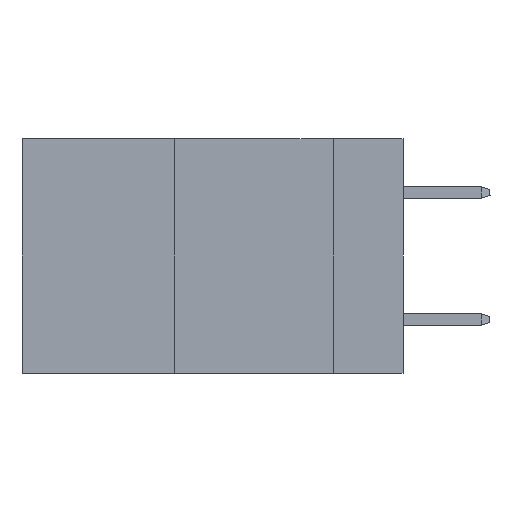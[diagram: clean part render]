
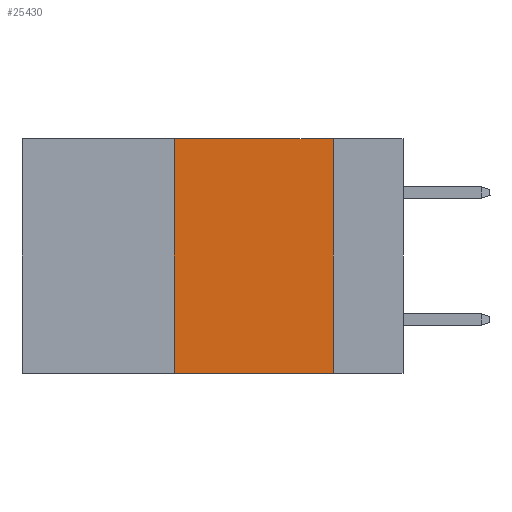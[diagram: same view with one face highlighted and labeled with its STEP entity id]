
A CAD part, left-side view. The second image highlights one B-rep face of the part: STEP entity #25430.
In plain terms, the highlighted planar face has unit normal (-1, 0, 0).
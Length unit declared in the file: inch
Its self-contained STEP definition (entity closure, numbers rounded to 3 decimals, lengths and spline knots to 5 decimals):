
#1773 = DIRECTION ( 'NONE',  ( 0., 0., -1. ) ) ;
#2760 = ORIENTED_EDGE ( 'NONE', *, *, #5335, .F. ) ;
#2932 = DIRECTION ( 'NONE',  ( 0., 0., -1. ) ) ;
#3067 = VERTEX_POINT ( 'NONE', #12259 ) ;
#4160 = EDGE_LOOP ( 'NONE', ( #13721, #2760, #11276, #19902 ) ) ;
#4776 = PLANE ( 'NONE',  #11750 ) ;
#4969 = DIRECTION ( 'NONE',  ( 1., 0., 0. ) ) ;
#5335 = EDGE_CURVE ( 'NONE', #18924, #26690, #37668, .T. ) ;
#7406 = VECTOR ( 'NONE', #2932, 39.37008 ) ;
#7564 = CARTESIAN_POINT ( 'NONE',  ( 0., 0.6, 0. ) ) ;
#8530 = LINE ( 'NONE', #23609, #27227 ) ;
#11276 = ORIENTED_EDGE ( 'NONE', *, *, #21764, .F. ) ;
#11750 = AXIS2_PLACEMENT_3D ( 'NONE', #7564, #4969, #1773 ) ;
#12259 = CARTESIAN_POINT ( 'NONE',  ( 0., 0.36, -0.37 ) ) ;
#13721 = ORIENTED_EDGE ( 'NONE', *, *, #30276, .F. ) ;
#14025 = LINE ( 'NONE', #23484, #18500 ) ;
#18130 = LINE ( 'NONE', #27776, #7406 ) ;
#18500 = VECTOR ( 'NONE', #23882, 39.37008 ) ;
#18924 = VERTEX_POINT ( 'NONE', #23296 ) ;
#19902 = ORIENTED_EDGE ( 'NONE', *, *, #28726, .T. ) ;
#20769 = CARTESIAN_POINT ( 'NONE',  ( 0., 0.11, -0.37 ) ) ;
#21764 = EDGE_CURVE ( 'NONE', #3067, #18924, #14025, .T. ) ;
#22200 = CARTESIAN_POINT ( 'NONE',  ( 0., 0.11, 0. ) ) ;
#22401 = CARTESIAN_POINT ( 'NONE',  ( 0., 0.6, 0. ) ) ;
#23296 = CARTESIAN_POINT ( 'NONE',  ( 0., 0.36, 0. ) ) ;
#23484 = CARTESIAN_POINT ( 'NONE',  ( 0., 0.36, 0. ) ) ;
#23609 = CARTESIAN_POINT ( 'NONE',  ( 0., 0.6, -0.37 ) ) ;
#23882 = DIRECTION ( 'NONE',  ( 0., 0., 1. ) ) ;
#25430 = ADVANCED_FACE ( 'NONE', ( #35075 ), #4776, .F. ) ;
#26690 = VERTEX_POINT ( 'NONE', #22200 ) ;
#27227 = VECTOR ( 'NONE', #35809, 39.37008 ) ;
#27776 = CARTESIAN_POINT ( 'NONE',  ( 0., 0.11, 0. ) ) ;
#28439 = VECTOR ( 'NONE', #31640, 39.37008 ) ;
#28726 = EDGE_CURVE ( 'NONE', #3067, #30217, #8530, .T. ) ;
#30217 = VERTEX_POINT ( 'NONE', #20769 ) ;
#30276 = EDGE_CURVE ( 'NONE', #26690, #30217, #18130, .T. ) ;
#31640 = DIRECTION ( 'NONE',  ( 0., -1., 0. ) ) ;
#35075 = FACE_OUTER_BOUND ( 'NONE', #4160, .T. ) ;
#35809 = DIRECTION ( 'NONE',  ( 0., -1., 0. ) ) ;
#37668 = LINE ( 'NONE', #22401, #28439 ) ;
